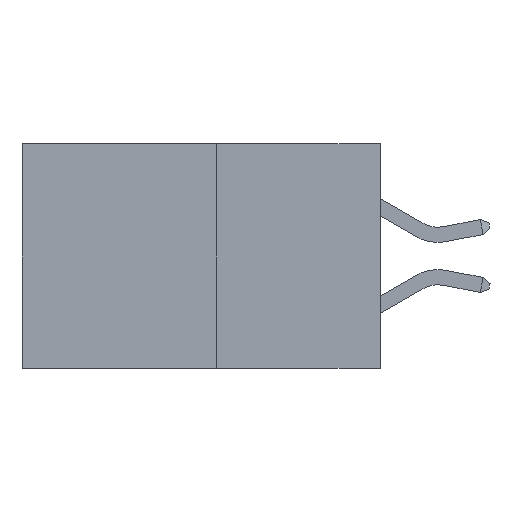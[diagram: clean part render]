
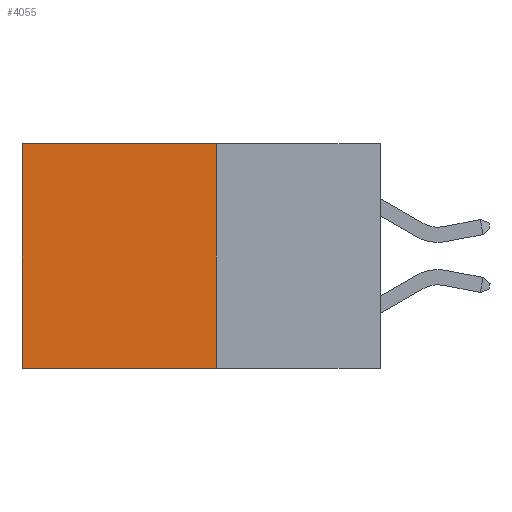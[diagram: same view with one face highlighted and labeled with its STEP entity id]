
A CAD part, left-side view. The second image highlights one B-rep face of the part: STEP entity #4055.
In plain terms, the highlighted planar face has unit normal (-1, 0, 0).
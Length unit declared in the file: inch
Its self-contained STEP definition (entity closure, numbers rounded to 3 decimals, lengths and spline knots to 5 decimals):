
#146 = DIRECTION ( 'NONE',  ( 0., 1., 0. ) ) ;
#207 = ORIENTED_EDGE ( 'NONE', *, *, #21284, .T. ) ;
#302 = LINE ( 'NONE', #10150, #21984 ) ;
#455 = CARTESIAN_POINT ( 'NONE',  ( 0.277, 0.27, 0. ) ) ;
#500 = CARTESIAN_POINT ( 'NONE',  ( 0.277, 0.27, -0.37 ) ) ;
#818 = DIRECTION ( 'NONE',  ( 0., 1., 0. ) ) ;
#1615 = DIRECTION ( 'NONE',  ( 0., 0., -1. ) ) ;
#2156 = DIRECTION ( 'NONE',  ( 0., 0., -1. ) ) ;
#4055 = ADVANCED_FACE ( 'NONE', ( #6828 ), #17026, .F. ) ;
#5305 = ORIENTED_EDGE ( 'NONE', *, *, #20358, .F. ) ;
#5481 = VECTOR ( 'NONE', #2156, 39.37008 ) ;
#6828 = FACE_OUTER_BOUND ( 'NONE', #13107, .T. ) ;
#7745 = ORIENTED_EDGE ( 'NONE', *, *, #8619, .F. ) ;
#8131 = ORIENTED_EDGE ( 'NONE', *, *, #19872, .T. ) ;
#8305 = LINE ( 'NONE', #455, #13427 ) ;
#8479 = DIRECTION ( 'NONE',  ( 0., 0., -1. ) ) ;
#8619 = EDGE_CURVE ( 'NONE', #9581, #14099, #20070, .T. ) ;
#9581 = VERTEX_POINT ( 'NONE', #500 ) ;
#9817 = VERTEX_POINT ( 'NONE', #18237 ) ;
#10150 = CARTESIAN_POINT ( 'NONE',  ( 0.277, 0.27, -0.37 ) ) ;
#10703 = CARTESIAN_POINT ( 'NONE',  ( 0.277, 0.59, -0.37 ) ) ;
#12805 = CARTESIAN_POINT ( 'NONE',  ( 0.277, 0.27, -0.37 ) ) ;
#13107 = EDGE_LOOP ( 'NONE', ( #8131, #7745, #5305, #207 ) ) ;
#13427 = VECTOR ( 'NONE', #146, 39.37008 ) ;
#14099 = VERTEX_POINT ( 'NONE', #16000 ) ;
#14500 = VECTOR ( 'NONE', #818, 39.37008 ) ;
#14604 = LINE ( 'NONE', #10703, #5481 ) ;
#15259 = CARTESIAN_POINT ( 'NONE',  ( 0.277, 0.27, -0.37 ) ) ;
#16000 = CARTESIAN_POINT ( 'NONE',  ( 0.277, 0.59, -0.37 ) ) ;
#16390 = VERTEX_POINT ( 'NONE', #17849 ) ;
#17026 = PLANE ( 'NONE',  #20041 ) ;
#17849 = CARTESIAN_POINT ( 'NONE',  ( 0.277, 0.59, 0. ) ) ;
#18237 = CARTESIAN_POINT ( 'NONE',  ( 0.277, 0.27, 0. ) ) ;
#18746 = DIRECTION ( 'NONE',  ( 1., 0., 0. ) ) ;
#19872 = EDGE_CURVE ( 'NONE', #16390, #14099, #14604, .T. ) ;
#20041 = AXIS2_PLACEMENT_3D ( 'NONE', #15259, #18746, #8479 ) ;
#20070 = LINE ( 'NONE', #12805, #14500 ) ;
#20358 = EDGE_CURVE ( 'NONE', #9817, #9581, #302, .T. ) ;
#21284 = EDGE_CURVE ( 'NONE', #9817, #16390, #8305, .T. ) ;
#21984 = VECTOR ( 'NONE', #1615, 39.37008 ) ;
